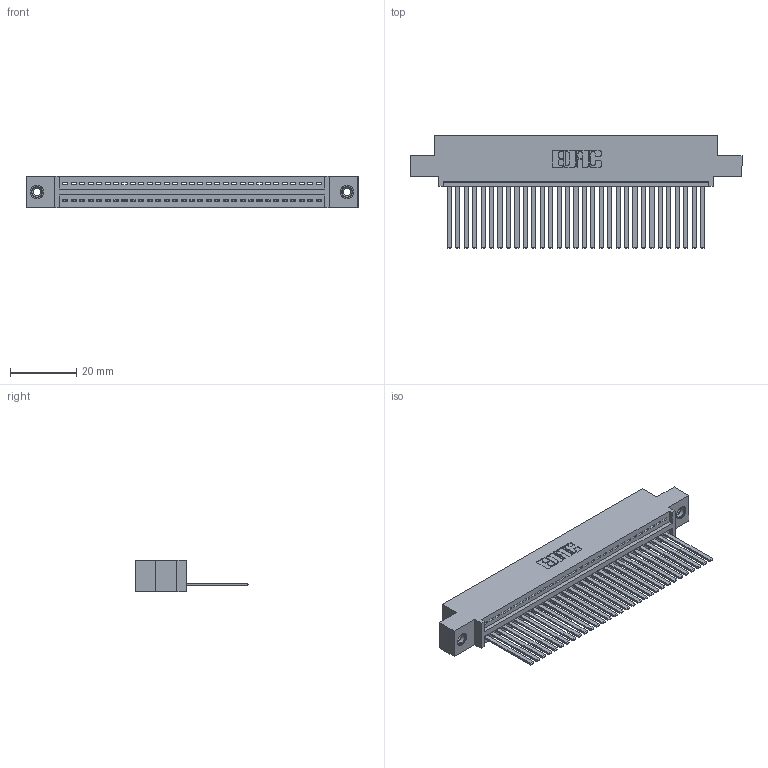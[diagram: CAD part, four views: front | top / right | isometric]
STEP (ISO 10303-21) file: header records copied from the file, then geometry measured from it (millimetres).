
FILE_DESCRIPTION (( 'STEP AP203' ), '1' );
FILE_NAME ('345-031-544-408.STEP', '2018-08-23T11:33:57', ( '' ), ( '' ), 'SwSTEP 2.0', 'SolidWorks 2016', '' );
FILE_SCHEMA (( 'CONFIG_CONTROL_DESIGN' ));
Length unit declared in the file: inch
Products named in the file (4): 345-292-001_345-293-144; 345-250-001_345-250-003-102; 345-031-544-408; 345 Part_0.110 Offset - 0.156 Dia-TI
Assembly tree (34 placements, depth 2):
  345-031-544-408
    345 Part_0.110 Offset - 0.156 Dia-TI
    345-292-001_345-293-144  x31
    345-250-001_345-250-003-102  x2
Bounding box: 99.95 x 33.96 x 9.4 mm (x, y, z)
Volume: 9682.3 mm3; surface area: 13896.2 mm2
Topology: 34 solids, 34 shells, 1802 faces, 5387 edges, 3542 vertices
Faces by surface type: plane 1232, cylinder 554, cone 12, torus 4
Entity records: 25946 total; most frequent: CARTESIAN_POINT 4476, ORIENTED_EDGE 4434, DIRECTION 3949, EDGE_CURVE 2217, VECTOR 1945, LINE 1945, VERTEX_POINT 1472, AXIS2_PLACEMENT_3D 1002
